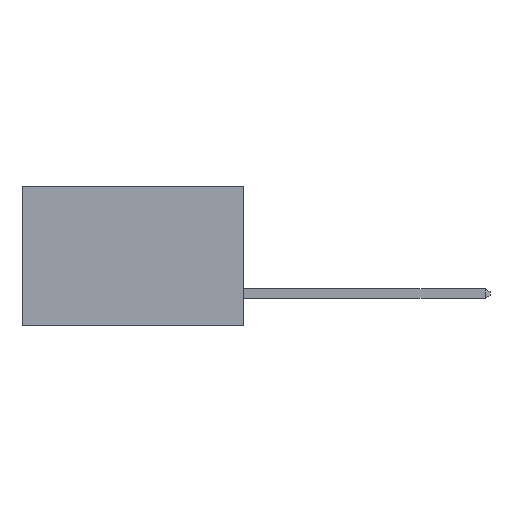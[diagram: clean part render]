
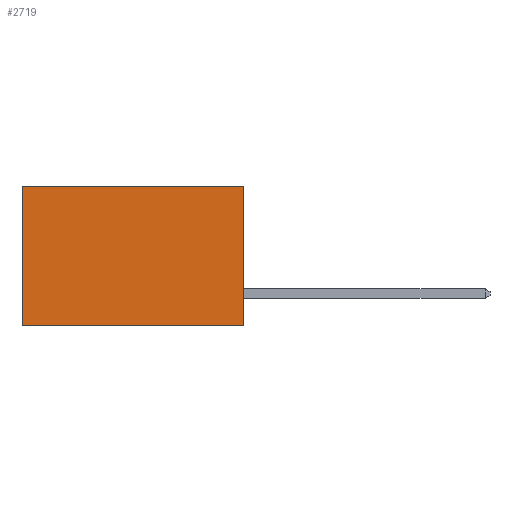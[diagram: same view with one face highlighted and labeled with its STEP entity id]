
A CAD part, left-side view. The second image highlights one B-rep face of the part: STEP entity #2719.
In plain terms, the highlighted planar face has unit normal (-1, 0, 0).
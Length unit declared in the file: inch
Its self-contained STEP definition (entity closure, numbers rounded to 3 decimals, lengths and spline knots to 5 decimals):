
#730 = ORIENTED_EDGE ( 'NONE', *, *, #9556, .F. ) ;
#979 = ORIENTED_EDGE ( 'NONE', *, *, #6127, .F. ) ;
#1200 = VECTOR ( 'NONE', #4958, 39.37008 ) ;
#1489 = VERTEX_POINT ( 'NONE', #6255 ) ;
#1814 = ORIENTED_EDGE ( 'NONE', *, *, #6998, .T. ) ;
#1815 = FACE_OUTER_BOUND ( 'NONE', #8942, .T. ) ;
#2506 = DIRECTION ( 'NONE',  ( 0., 0., -1. ) ) ;
#2548 = DIRECTION ( 'NONE',  ( 0., 0., -1. ) ) ;
#2719 = ADVANCED_FACE ( 'NONE', ( #1815 ), #5098, .F. ) ;
#3155 = AXIS2_PLACEMENT_3D ( 'NONE', #6867, #7591, #2548 ) ;
#3257 = LINE ( 'NONE', #7831, #6997 ) ;
#4154 = CARTESIAN_POINT ( 'NONE',  ( 0.277, 0., -0.37 ) ) ;
#4279 = CARTESIAN_POINT ( 'NONE',  ( 0.277, 0., 0. ) ) ;
#4306 = VECTOR ( 'NONE', #2506, 39.37008 ) ;
#4543 = LINE ( 'NONE', #9211, #4306 ) ;
#4790 = DIRECTION ( 'NONE',  ( 0., 0., -1. ) ) ;
#4958 = DIRECTION ( 'NONE',  ( 0., 1., 0. ) ) ;
#5029 = ORIENTED_EDGE ( 'NONE', *, *, #9445, .T. ) ;
#5098 = PLANE ( 'NONE',  #3155 ) ;
#5607 = LINE ( 'NONE', #7011, #9254 ) ;
#5682 = VERTEX_POINT ( 'NONE', #7384 ) ;
#6127 = EDGE_CURVE ( 'NONE', #8811, #1489, #3257, .T. ) ;
#6255 = CARTESIAN_POINT ( 'NONE',  ( 0.277, 0., -0.37 ) ) ;
#6270 = DIRECTION ( 'NONE',  ( 0., 1., 0. ) ) ;
#6867 = CARTESIAN_POINT ( 'NONE',  ( 0.277, 0., -0.37 ) ) ;
#6997 = VECTOR ( 'NONE', #4790, 39.37008 ) ;
#6998 = EDGE_CURVE ( 'NONE', #8811, #5682, #5607, .T. ) ;
#7011 = CARTESIAN_POINT ( 'NONE',  ( 0.277, 0., 0. ) ) ;
#7285 = CARTESIAN_POINT ( 'NONE',  ( 0.277, 0.59, -0.37 ) ) ;
#7291 = LINE ( 'NONE', #4154, #1200 ) ;
#7384 = CARTESIAN_POINT ( 'NONE',  ( 0.277, 0.59, 0. ) ) ;
#7591 = DIRECTION ( 'NONE',  ( 1., 0., 0. ) ) ;
#7831 = CARTESIAN_POINT ( 'NONE',  ( 0.277, 0., -0.37 ) ) ;
#8811 = VERTEX_POINT ( 'NONE', #4279 ) ;
#8942 = EDGE_LOOP ( 'NONE', ( #5029, #730, #979, #1814 ) ) ;
#9211 = CARTESIAN_POINT ( 'NONE',  ( 0.277, 0.59, -0.37 ) ) ;
#9254 = VECTOR ( 'NONE', #6270, 39.37008 ) ;
#9445 = EDGE_CURVE ( 'NONE', #5682, #9743, #4543, .T. ) ;
#9556 = EDGE_CURVE ( 'NONE', #1489, #9743, #7291, .T. ) ;
#9743 = VERTEX_POINT ( 'NONE', #7285 ) ;
